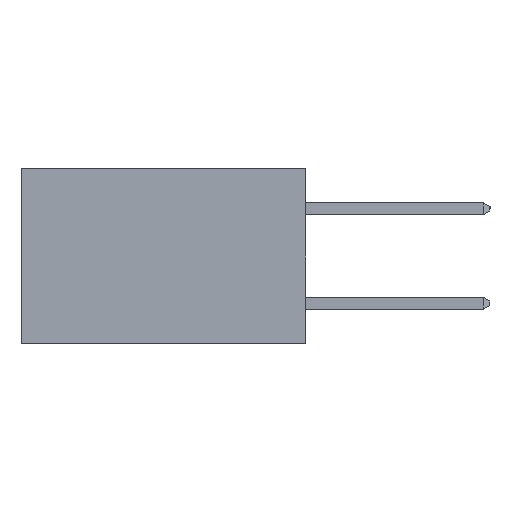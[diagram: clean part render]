
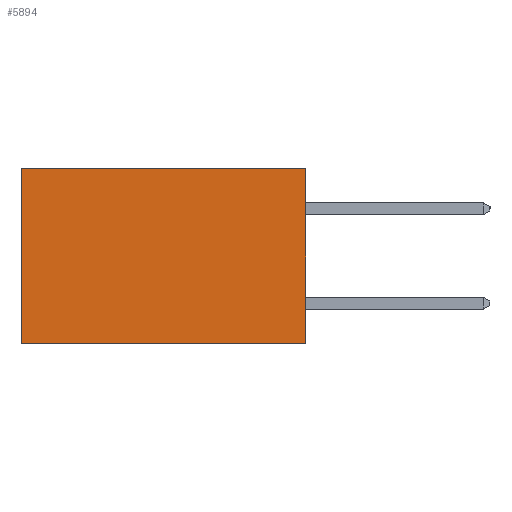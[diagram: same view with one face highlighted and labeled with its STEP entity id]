
A CAD part, left-side view. The second image highlights one B-rep face of the part: STEP entity #5894.
In plain terms, the highlighted planar face has unit normal (-1, 0, 0).
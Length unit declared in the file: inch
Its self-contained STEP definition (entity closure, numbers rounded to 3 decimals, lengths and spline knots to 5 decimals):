
#129 = VECTOR ( 'NONE', #5301, 39.37008 ) ;
#418 = CARTESIAN_POINT ( 'NONE',  ( 0.2615, 0.6, -0.37 ) ) ;
#832 = ORIENTED_EDGE ( 'NONE', *, *, #1046, .F. ) ;
#911 = LINE ( 'NONE', #19144, #9959 ) ;
#1046 = EDGE_CURVE ( 'NONE', #14518, #1819, #911, .T. ) ;
#1457 = VERTEX_POINT ( 'NONE', #9744 ) ;
#1711 = ORIENTED_EDGE ( 'NONE', *, *, #11849, .T. ) ;
#1819 = VERTEX_POINT ( 'NONE', #16964 ) ;
#2042 = DIRECTION ( 'NONE',  ( 0., 1., 0. ) ) ;
#2985 = DIRECTION ( 'NONE',  ( 0., 0., -1. ) ) ;
#3456 = DIRECTION ( 'NONE',  ( 0., 0., -1. ) ) ;
#3581 = CARTESIAN_POINT ( 'NONE',  ( 0.2615, 0., 0. ) ) ;
#3918 = DIRECTION ( 'NONE',  ( 0., 0., -1. ) ) ;
#4516 = VECTOR ( 'NONE', #3456, 39.37008 ) ;
#5301 = DIRECTION ( 'NONE',  ( 0., 1., 0. ) ) ;
#5894 = ADVANCED_FACE ( 'NONE', ( #7559 ), #13795, .F. ) ;
#7559 = FACE_OUTER_BOUND ( 'NONE', #17915, .T. ) ;
#8060 = LINE ( 'NONE', #17532, #129 ) ;
#9599 = VECTOR ( 'NONE', #3918, 39.37008 ) ;
#9744 = CARTESIAN_POINT ( 'NONE',  ( 0.2615, 0.6, 0. ) ) ;
#9959 = VECTOR ( 'NONE', #2042, 39.37008 ) ;
#10097 = VERTEX_POINT ( 'NONE', #3581 ) ;
#11681 = LINE ( 'NONE', #19296, #9599 ) ;
#11849 = EDGE_CURVE ( 'NONE', #1457, #1819, #17814, .T. ) ;
#12275 = DIRECTION ( 'NONE',  ( 1., 0., 0. ) ) ;
#12676 = AXIS2_PLACEMENT_3D ( 'NONE', #19983, #12275, #2985 ) ;
#13795 = PLANE ( 'NONE',  #12676 ) ;
#14518 = VERTEX_POINT ( 'NONE', #15582 ) ;
#15582 = CARTESIAN_POINT ( 'NONE',  ( 0.2615, 0., -0.37 ) ) ;
#16783 = EDGE_CURVE ( 'NONE', #10097, #1457, #8060, .T. ) ;
#16964 = CARTESIAN_POINT ( 'NONE',  ( 0.2615, 0.6, -0.37 ) ) ;
#17182 = ORIENTED_EDGE ( 'NONE', *, *, #16783, .T. ) ;
#17289 = ORIENTED_EDGE ( 'NONE', *, *, #19320, .F. ) ;
#17532 = CARTESIAN_POINT ( 'NONE',  ( 0.2615, 0., 0. ) ) ;
#17814 = LINE ( 'NONE', #418, #4516 ) ;
#17915 = EDGE_LOOP ( 'NONE', ( #1711, #832, #17289, #17182 ) ) ;
#19144 = CARTESIAN_POINT ( 'NONE',  ( 0.2615, 0., -0.37 ) ) ;
#19296 = CARTESIAN_POINT ( 'NONE',  ( 0.2615, 0., -0.37 ) ) ;
#19320 = EDGE_CURVE ( 'NONE', #10097, #14518, #11681, .T. ) ;
#19983 = CARTESIAN_POINT ( 'NONE',  ( 0.2615, 0., -0.37 ) ) ;
